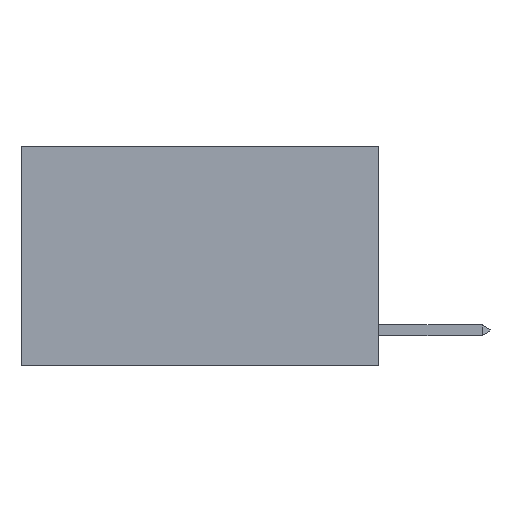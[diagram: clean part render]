
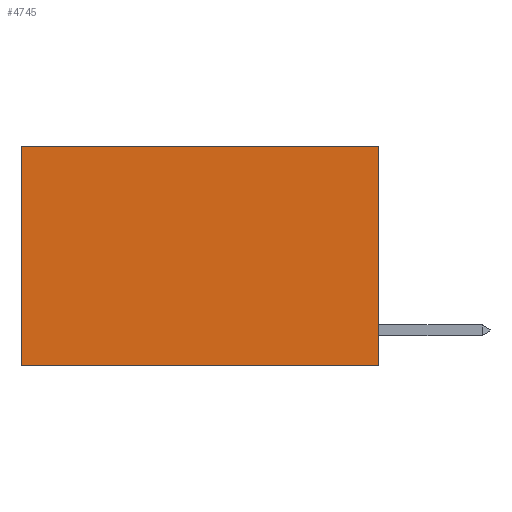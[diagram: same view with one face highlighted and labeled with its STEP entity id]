
A CAD part, left-side view. The second image highlights one B-rep face of the part: STEP entity #4745.
In plain terms, the highlighted planar face has unit normal (-1, 0, 0).
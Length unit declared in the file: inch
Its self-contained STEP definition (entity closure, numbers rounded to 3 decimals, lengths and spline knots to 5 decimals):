
#317 = ORIENTED_EDGE ( 'NONE', *, *, #11454, .F. ) ;
#1094 = VERTEX_POINT ( 'NONE', #4577 ) ;
#2456 = EDGE_CURVE ( 'NONE', #7435, #4479, #18576, .T. ) ;
#3100 = ORIENTED_EDGE ( 'NONE', *, *, #2456, .T. ) ;
#3176 = DIRECTION ( 'NONE',  ( 0., 1., 0. ) ) ;
#3412 = CARTESIAN_POINT ( 'NONE',  ( 0.2625, 0., 0. ) ) ;
#3440 = EDGE_LOOP ( 'NONE', ( #14662, #317, #13504, #3100 ) ) ;
#3458 = VECTOR ( 'NONE', #3176, 39.37008 ) ;
#3968 = CARTESIAN_POINT ( 'NONE',  ( 0.2625, 0., 0. ) ) ;
#4055 = EDGE_CURVE ( 'NONE', #4479, #7347, #17433, .T. ) ;
#4479 = VERTEX_POINT ( 'NONE', #11725 ) ;
#4577 = CARTESIAN_POINT ( 'NONE',  ( 0.2625, 0., -0.37 ) ) ;
#4745 = ADVANCED_FACE ( 'NONE', ( #16772 ), #11048, .F. ) ;
#4853 = DIRECTION ( 'NONE',  ( 0., 0., -1. ) ) ;
#6525 = LINE ( 'NONE', #15137, #13750 ) ;
#6682 = DIRECTION ( 'NONE',  ( 0., 0., -1. ) ) ;
#7347 = VERTEX_POINT ( 'NONE', #11122 ) ;
#7435 = VERTEX_POINT ( 'NONE', #9831 ) ;
#7875 = AXIS2_PLACEMENT_3D ( 'NONE', #13869, #15295, #6682 ) ;
#9831 = CARTESIAN_POINT ( 'NONE',  ( 0.2625, 0., 0. ) ) ;
#10752 = VECTOR ( 'NONE', #4853, 39.37008 ) ;
#11048 = PLANE ( 'NONE',  #7875 ) ;
#11122 = CARTESIAN_POINT ( 'NONE',  ( 0.2625, 0.6, -0.37 ) ) ;
#11210 = LINE ( 'NONE', #3412, #10752 ) ;
#11454 = EDGE_CURVE ( 'NONE', #1094, #7347, #6525, .T. ) ;
#11725 = CARTESIAN_POINT ( 'NONE',  ( 0.2625, 0.6, 0. ) ) ;
#13259 = VECTOR ( 'NONE', #17929, 39.37008 ) ;
#13504 = ORIENTED_EDGE ( 'NONE', *, *, #16167, .F. ) ;
#13750 = VECTOR ( 'NONE', #17931, 39.37008 ) ;
#13869 = CARTESIAN_POINT ( 'NONE',  ( 0.2625, 0., 0. ) ) ;
#14662 = ORIENTED_EDGE ( 'NONE', *, *, #4055, .T. ) ;
#15137 = CARTESIAN_POINT ( 'NONE',  ( 0.2625, 0., -0.37 ) ) ;
#15295 = DIRECTION ( 'NONE',  ( 1., 0., 0. ) ) ;
#16167 = EDGE_CURVE ( 'NONE', #7435, #1094, #11210, .T. ) ;
#16538 = CARTESIAN_POINT ( 'NONE',  ( 0.2625, 0.6, 0. ) ) ;
#16772 = FACE_OUTER_BOUND ( 'NONE', #3440, .T. ) ;
#17433 = LINE ( 'NONE', #16538, #13259 ) ;
#17929 = DIRECTION ( 'NONE',  ( 0., 0., -1. ) ) ;
#17931 = DIRECTION ( 'NONE',  ( 0., 1., 0. ) ) ;
#18576 = LINE ( 'NONE', #3968, #3458 ) ;
